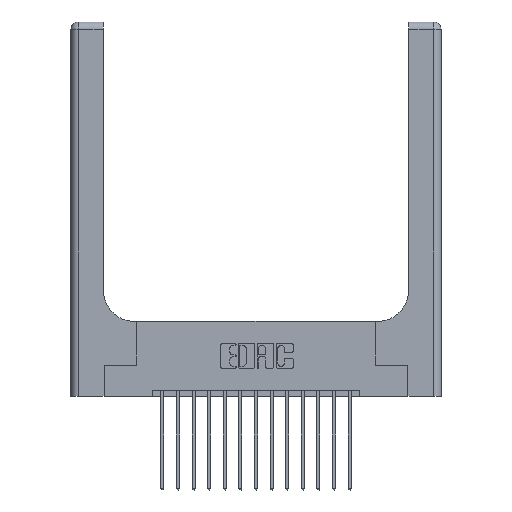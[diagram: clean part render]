
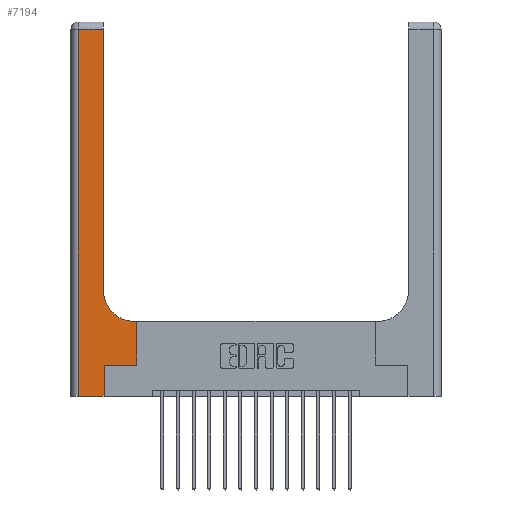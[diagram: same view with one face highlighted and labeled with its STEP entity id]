
A CAD part, top view. The second image highlights one B-rep face of the part: STEP entity #7194.
In plain terms, the highlighted planar face has unit normal (0, 0, 1).
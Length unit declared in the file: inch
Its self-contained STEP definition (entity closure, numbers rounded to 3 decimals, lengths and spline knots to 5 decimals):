
#824 = VERTEX_POINT ( 'NONE', #7976 ) ;
#951 = DIRECTION ( 'NONE',  ( 0., 1., 0. ) ) ;
#1148 = LINE ( 'NONE', #6511, #16882 ) ;
#1371 = VERTEX_POINT ( 'NONE', #10364 ) ;
#1623 = DIRECTION ( 'NONE',  ( 0., -1., 0. ) ) ;
#2014 = EDGE_LOOP ( 'NONE', ( #12258, #10312, #16767, #11356, #15910, #7808, #5925, #10075, #3430 ) ) ;
#2193 = DIRECTION ( 'NONE',  ( 0., 0., -1. ) ) ;
#2209 = AXIS2_PLACEMENT_3D ( 'NONE', #12841, #11311, #7204 ) ;
#2298 = CARTESIAN_POINT ( 'NONE',  ( 0.26, 2.94, 0.37 ) ) ;
#2726 = DIRECTION ( 'NONE',  ( 1., 0., 0. ) ) ;
#3120 = VERTEX_POINT ( 'NONE', #15648 ) ;
#3430 = ORIENTED_EDGE ( 'NONE', *, *, #4755, .T. ) ;
#4365 = CARTESIAN_POINT ( 'NONE',  ( 0.06, 0., 0.37 ) ) ;
#4501 = VECTOR ( 'NONE', #1623, 39.37008 ) ;
#4512 = VERTEX_POINT ( 'NONE', #16418 ) ;
#4755 = EDGE_CURVE ( 'NONE', #7953, #3120, #5419, .T. ) ;
#4814 = EDGE_CURVE ( 'NONE', #1371, #7953, #17298, .T. ) ;
#4934 = AXIS2_PLACEMENT_3D ( 'NONE', #12985, #2193, #13050 ) ;
#4997 = DIRECTION ( 'NONE',  ( -1., 0., 0. ) ) ;
#4998 = DIRECTION ( 'NONE',  ( -1., 0., 0. ) ) ;
#5028 = VERTEX_POINT ( 'NONE', #4365 ) ;
#5419 = CIRCLE ( 'NONE', #4934, 0.25 ) ;
#5925 = ORIENTED_EDGE ( 'NONE', *, *, #17319, .T. ) ;
#6225 = CARTESIAN_POINT ( 'NONE',  ( 0.51, 0.6, 0.37 ) ) ;
#6361 = EDGE_CURVE ( 'NONE', #12435, #824, #7510, .T. ) ;
#6511 = CARTESIAN_POINT ( 'NONE',  ( 0., 2.94, 0.37 ) ) ;
#6946 = EDGE_CURVE ( 'NONE', #12961, #12435, #13677, .T. ) ;
#7194 = ADVANCED_FACE ( 'NONE', ( #11518 ), #16842, .F. ) ;
#7204 = DIRECTION ( 'NONE',  ( -1., 0., 0. ) ) ;
#7509 = LINE ( 'NONE', #11065, #4501 ) ;
#7510 = LINE ( 'NONE', #14864, #11746 ) ;
#7808 = ORIENTED_EDGE ( 'NONE', *, *, #6361, .T. ) ;
#7910 = DIRECTION ( 'NONE',  ( 1., 0., 0. ) ) ;
#7953 = VERTEX_POINT ( 'NONE', #6225 ) ;
#7976 = CARTESIAN_POINT ( 'NONE',  ( 0.528, 0.25, 0.37 ) ) ;
#8077 = LINE ( 'NONE', #11800, #12295 ) ;
#9348 = CARTESIAN_POINT ( 'NONE',  ( 0., 0., 0.37 ) ) ;
#9880 = VECTOR ( 'NONE', #11144, 39.37008 ) ;
#10075 = ORIENTED_EDGE ( 'NONE', *, *, #4814, .T. ) ;
#10312 = ORIENTED_EDGE ( 'NONE', *, *, #11288, .T. ) ;
#10340 = CARTESIAN_POINT ( 'NONE',  ( 0.26, 0.6, 0.37 ) ) ;
#10364 = CARTESIAN_POINT ( 'NONE',  ( 0.528, 0.6, 0.37 ) ) ;
#10538 = CARTESIAN_POINT ( 'NONE',  ( 0.26, 3., 0.37 ) ) ;
#10653 = DIRECTION ( 'NONE',  ( 0., 1., 0. ) ) ;
#11065 = CARTESIAN_POINT ( 'NONE',  ( 0.06, 3., 0.37 ) ) ;
#11086 = LINE ( 'NONE', #9348, #13195 ) ;
#11144 = DIRECTION ( 'NONE',  ( 0., 1., 0. ) ) ;
#11288 = EDGE_CURVE ( 'NONE', #15870, #4512, #1148, .T. ) ;
#11311 = DIRECTION ( 'NONE',  ( 0., 0., -1. ) ) ;
#11356 = ORIENTED_EDGE ( 'NONE', *, *, #16606, .T. ) ;
#11518 = FACE_OUTER_BOUND ( 'NONE', #2014, .T. ) ;
#11746 = VECTOR ( 'NONE', #2726, 39.37008 ) ;
#11800 = CARTESIAN_POINT ( 'NONE',  ( 0.528, 0.25, 0.37 ) ) ;
#11922 = LINE ( 'NONE', #10538, #15275 ) ;
#12258 = ORIENTED_EDGE ( 'NONE', *, *, #16711, .T. ) ;
#12295 = VECTOR ( 'NONE', #951, 39.37008 ) ;
#12303 = CARTESIAN_POINT ( 'NONE',  ( 0.265, 0., 0.37 ) ) ;
#12435 = VERTEX_POINT ( 'NONE', #16509 ) ;
#12841 = CARTESIAN_POINT ( 'NONE',  ( 0., 3., 0.37 ) ) ;
#12961 = VERTEX_POINT ( 'NONE', #16552 ) ;
#12985 = CARTESIAN_POINT ( 'NONE',  ( 0.51, 0.85, 0.37 ) ) ;
#13050 = DIRECTION ( 'NONE',  ( 1., 0., 0. ) ) ;
#13195 = VECTOR ( 'NONE', #7910, 39.37008 ) ;
#13553 = EDGE_CURVE ( 'NONE', #4512, #5028, #7509, .T. ) ;
#13677 = LINE ( 'NONE', #12303, #9880 ) ;
#13710 = VECTOR ( 'NONE', #4997, 39.37008 ) ;
#14864 = CARTESIAN_POINT ( 'NONE',  ( 0.265, 0.25, 0.37 ) ) ;
#15275 = VECTOR ( 'NONE', #10653, 39.37008 ) ;
#15648 = CARTESIAN_POINT ( 'NONE',  ( 0.26, 0.85, 0.37 ) ) ;
#15870 = VERTEX_POINT ( 'NONE', #2298 ) ;
#15910 = ORIENTED_EDGE ( 'NONE', *, *, #6946, .T. ) ;
#16418 = CARTESIAN_POINT ( 'NONE',  ( 0.06, 2.94, 0.37 ) ) ;
#16509 = CARTESIAN_POINT ( 'NONE',  ( 0.265, 0.25, 0.37 ) ) ;
#16552 = CARTESIAN_POINT ( 'NONE',  ( 0.265, 0., 0.37 ) ) ;
#16606 = EDGE_CURVE ( 'NONE', #5028, #12961, #11086, .T. ) ;
#16711 = EDGE_CURVE ( 'NONE', #3120, #15870, #11922, .T. ) ;
#16767 = ORIENTED_EDGE ( 'NONE', *, *, #13553, .T. ) ;
#16842 = PLANE ( 'NONE',  #2209 ) ;
#16882 = VECTOR ( 'NONE', #4998, 39.37008 ) ;
#17298 = LINE ( 'NONE', #10340, #13710 ) ;
#17319 = EDGE_CURVE ( 'NONE', #824, #1371, #8077, .T. ) ;
